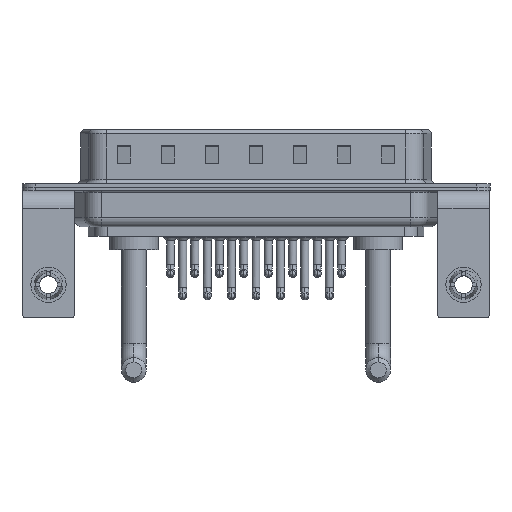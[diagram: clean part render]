
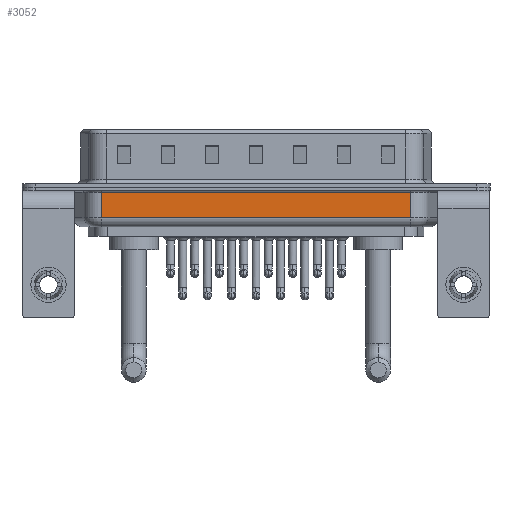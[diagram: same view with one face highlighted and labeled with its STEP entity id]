
A CAD part, front view. The second image highlights one B-rep face of the part: STEP entity #3052.
In plain terms, the highlighted planar face has unit normal (0, -1, 0).
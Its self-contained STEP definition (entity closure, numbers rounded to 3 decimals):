
#196 = ORIENTED_EDGE ( 'NONE', *, *, #11432, .F. ) ;
#335 = ORIENTED_EDGE ( 'NONE', *, *, #4381, .T. ) ;
#1009 = ORIENTED_EDGE ( 'NONE', *, *, #14054, .T. ) ;
#1147 = EDGE_LOOP ( 'NONE', ( #196, #335, #1009, #22081 ) ) ;
#1675 = DIRECTION ( 'NONE',  ( 0., 1., 0. ) ) ;
#2477 = VECTOR ( 'NONE', #14984, 1000. ) ;
#3052 = ADVANCED_FACE ( 'NONE', ( #23323 ), #22911, .F. ) ;
#3890 = DIRECTION ( 'NONE',  ( 0., 0., 1. ) ) ;
#4240 = CARTESIAN_POINT ( 'NONE',  ( 6.006, -5.35, -0.65 ) ) ;
#4381 = EDGE_CURVE ( 'NONE', #13321, #13649, #11934, .T. ) ;
#5308 = VERTEX_POINT ( 'NONE', #21604 ) ;
#6958 = VECTOR ( 'NONE', #24425, 1000. ) ;
#8668 = DIRECTION ( 'NONE',  ( -1., 0., 0. ) ) ;
#9753 = CARTESIAN_POINT ( 'NONE',  ( 41.044, -5.35, -3.5 ) ) ;
#10673 = VECTOR ( 'NONE', #8668, 1000. ) ;
#11432 = EDGE_CURVE ( 'NONE', #13321, #5308, #13561, .T. ) ;
#11577 = CARTESIAN_POINT ( 'NONE',  ( 6.006, -5.35, -3.5 ) ) ;
#11934 = LINE ( 'NONE', #18292, #16813 ) ;
#13321 = VERTEX_POINT ( 'NONE', #11577 ) ;
#13561 = LINE ( 'NONE', #22069, #6958 ) ;
#13649 = VERTEX_POINT ( 'NONE', #9753 ) ;
#14054 = EDGE_CURVE ( 'NONE', #13649, #18360, #17196, .T. ) ;
#14390 = CARTESIAN_POINT ( 'NONE',  ( 6.006, -5.35, -4.5 ) ) ;
#14984 = DIRECTION ( 'NONE',  ( 0., 0., 1. ) ) ;
#16813 = VECTOR ( 'NONE', #27259, 1000. ) ;
#17196 = LINE ( 'NONE', #19386, #2477 ) ;
#18292 = CARTESIAN_POINT ( 'NONE',  ( 6.006, -5.35, -3.5 ) ) ;
#18360 = VERTEX_POINT ( 'NONE', #21356 ) ;
#18862 = LINE ( 'NONE', #4240, #10673 ) ;
#19386 = CARTESIAN_POINT ( 'NONE',  ( 41.044, -5.35, -4.5 ) ) ;
#21278 = EDGE_CURVE ( 'NONE', #18360, #5308, #18862, .T. ) ;
#21356 = CARTESIAN_POINT ( 'NONE',  ( 41.044, -5.35, -0.65 ) ) ;
#21604 = CARTESIAN_POINT ( 'NONE',  ( 6.006, -5.35, -0.65 ) ) ;
#22069 = CARTESIAN_POINT ( 'NONE',  ( 6.006, -5.35, -4.5 ) ) ;
#22081 = ORIENTED_EDGE ( 'NONE', *, *, #21278, .T. ) ;
#22909 = AXIS2_PLACEMENT_3D ( 'NONE', #14390, #1675, #3890 ) ;
#22911 = PLANE ( 'NONE',  #22909 ) ;
#23323 = FACE_OUTER_BOUND ( 'NONE', #1147, .T. ) ;
#24425 = DIRECTION ( 'NONE',  ( 0., 0., 1. ) ) ;
#27259 = DIRECTION ( 'NONE',  ( 1., 0., 0. ) ) ;
